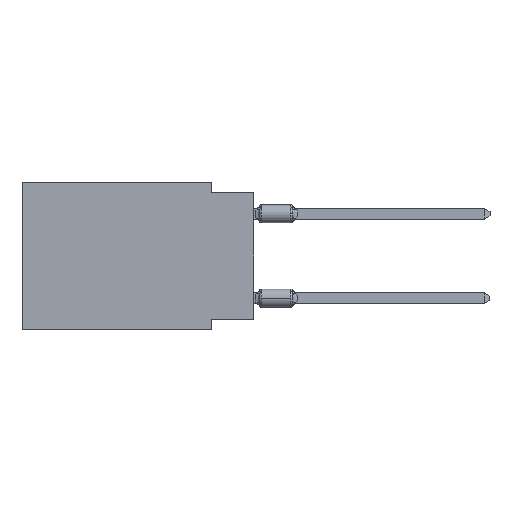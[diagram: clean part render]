
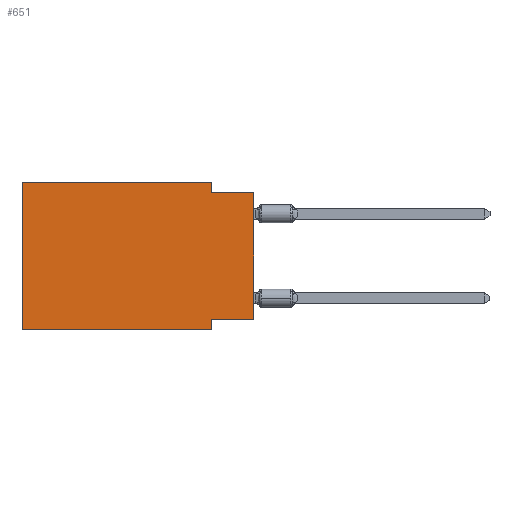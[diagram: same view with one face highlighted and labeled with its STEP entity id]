
A CAD part, left-side view. The second image highlights one B-rep face of the part: STEP entity #651.
In plain terms, the highlighted planar face has unit normal (-1, 0, 0).
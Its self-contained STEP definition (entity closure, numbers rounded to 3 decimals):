
#324 = LINE ( 'NONE', #16808, #6538 ) ;
#423 = ORIENTED_EDGE ( 'NONE', *, *, #13755, .F. ) ;
#651 = ADVANCED_FACE ( 'NONE', ( #12533 ), #8059, .F. ) ;
#663 = DIRECTION ( 'NONE',  ( 0., -1., 0. ) ) ;
#703 = ORIENTED_EDGE ( 'NONE', *, *, #3946, .F. ) ;
#1146 = VECTOR ( 'NONE', #19174, 1000. ) ;
#1623 = LINE ( 'NONE', #10760, #12921 ) ;
#2110 = ORIENTED_EDGE ( 'NONE', *, *, #7464, .T. ) ;
#2690 = VECTOR ( 'NONE', #2769, 1000. ) ;
#2769 = DIRECTION ( 'NONE',  ( 0., -1., 0. ) ) ;
#3230 = VERTEX_POINT ( 'NONE', #16482 ) ;
#3675 = EDGE_LOOP ( 'NONE', ( #2110, #6199, #4743, #703, #423, #17135, #8016, #7773 ) ) ;
#3909 = LINE ( 'NONE', #14442, #17292 ) ;
#3946 = EDGE_CURVE ( 'NONE', #7604, #10179, #15749, .T. ) ;
#4677 = VECTOR ( 'NONE', #16977, 1000. ) ;
#4743 = ORIENTED_EDGE ( 'NONE', *, *, #13432, .F. ) ;
#4866 = VECTOR ( 'NONE', #663, 1000. ) ;
#4951 = EDGE_CURVE ( 'NONE', #10436, #18415, #17949, .T. ) ;
#5174 = DIRECTION ( 'NONE',  ( 1., 0., 0. ) ) ;
#5371 = CARTESIAN_POINT ( 'NONE',  ( 0., 0., 0. ) ) ;
#6199 = ORIENTED_EDGE ( 'NONE', *, *, #4951, .F. ) ;
#6538 = VECTOR ( 'NONE', #16898, 1000. ) ;
#7009 = DIRECTION ( 'NONE',  ( 0., 0., -1. ) ) ;
#7039 = CARTESIAN_POINT ( 'NONE',  ( 0., 2.54, -0.635 ) ) ;
#7042 = EDGE_CURVE ( 'NONE', #18877, #3230, #1623, .T. ) ;
#7155 = DIRECTION ( 'NONE',  ( 0., -1., 0. ) ) ;
#7464 = EDGE_CURVE ( 'NONE', #17673, #18415, #14092, .T. ) ;
#7604 = VERTEX_POINT ( 'NONE', #16075 ) ;
#7773 = ORIENTED_EDGE ( 'NONE', *, *, #18128, .F. ) ;
#7943 = CARTESIAN_POINT ( 'NONE',  ( 0., 2.54, 0. ) ) ;
#8016 = ORIENTED_EDGE ( 'NONE', *, *, #7042, .F. ) ;
#8059 = PLANE ( 'NONE',  #15699 ) ;
#8087 = VECTOR ( 'NONE', #7155, 1000. ) ;
#8930 = CARTESIAN_POINT ( 'NONE',  ( 0., 13.97, -8.89 ) ) ;
#9033 = LINE ( 'NONE', #16180, #8087 ) ;
#9638 = CARTESIAN_POINT ( 'NONE',  ( 0., 2.54, -8.255 ) ) ;
#10179 = VERTEX_POINT ( 'NONE', #7943 ) ;
#10420 = CARTESIAN_POINT ( 'NONE',  ( 0., 0., -0.635 ) ) ;
#10436 = VERTEX_POINT ( 'NONE', #7039 ) ;
#10760 = CARTESIAN_POINT ( 'NONE',  ( 0., 2.54, -8.89 ) ) ;
#11708 = VERTEX_POINT ( 'NONE', #8930 ) ;
#12533 = FACE_OUTER_BOUND ( 'NONE', #3675, .T. ) ;
#12831 = DIRECTION ( 'NONE',  ( 0., 0., -1. ) ) ;
#12921 = VECTOR ( 'NONE', #16605, 1000. ) ;
#13121 = CARTESIAN_POINT ( 'NONE',  ( 0., 0., -8.255 ) ) ;
#13139 = CARTESIAN_POINT ( 'NONE',  ( 0., 0., -8.255 ) ) ;
#13432 = EDGE_CURVE ( 'NONE', #10179, #10436, #3909, .T. ) ;
#13755 = EDGE_CURVE ( 'NONE', #11708, #7604, #324, .T. ) ;
#14092 = LINE ( 'NONE', #5371, #4677 ) ;
#14191 = CARTESIAN_POINT ( 'NONE',  ( 0., 0., -0.635 ) ) ;
#14267 = CARTESIAN_POINT ( 'NONE',  ( 0., 13.97, 0. ) ) ;
#14442 = CARTESIAN_POINT ( 'NONE',  ( 0., 2.54, 0. ) ) ;
#14607 = LINE ( 'NONE', #13121, #1146 ) ;
#15699 = AXIS2_PLACEMENT_3D ( 'NONE', #18788, #5174, #12831 ) ;
#15749 = LINE ( 'NONE', #14267, #4866 ) ;
#16075 = CARTESIAN_POINT ( 'NONE',  ( 0., 13.97, 0. ) ) ;
#16180 = CARTESIAN_POINT ( 'NONE',  ( 0., 13.97, -8.89 ) ) ;
#16482 = CARTESIAN_POINT ( 'NONE',  ( 0., 2.54, -8.89 ) ) ;
#16605 = DIRECTION ( 'NONE',  ( 0., 0., -1. ) ) ;
#16808 = CARTESIAN_POINT ( 'NONE',  ( 0., 13.97, 0. ) ) ;
#16898 = DIRECTION ( 'NONE',  ( 0., 0., 1. ) ) ;
#16924 = EDGE_CURVE ( 'NONE', #11708, #3230, #9033, .T. ) ;
#16977 = DIRECTION ( 'NONE',  ( 0., 0., 1. ) ) ;
#17135 = ORIENTED_EDGE ( 'NONE', *, *, #16924, .T. ) ;
#17292 = VECTOR ( 'NONE', #7009, 1000. ) ;
#17673 = VERTEX_POINT ( 'NONE', #13139 ) ;
#17949 = LINE ( 'NONE', #10420, #2690 ) ;
#18128 = EDGE_CURVE ( 'NONE', #17673, #18877, #14607, .T. ) ;
#18415 = VERTEX_POINT ( 'NONE', #14191 ) ;
#18788 = CARTESIAN_POINT ( 'NONE',  ( 0., 13.97, 0. ) ) ;
#18877 = VERTEX_POINT ( 'NONE', #9638 ) ;
#19174 = DIRECTION ( 'NONE',  ( 0., 1., 0. ) ) ;
